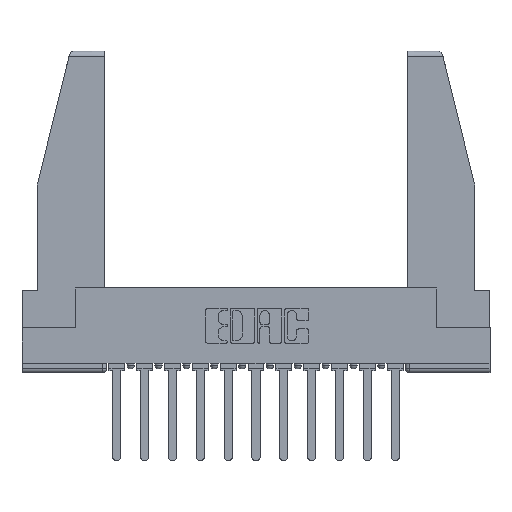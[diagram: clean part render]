
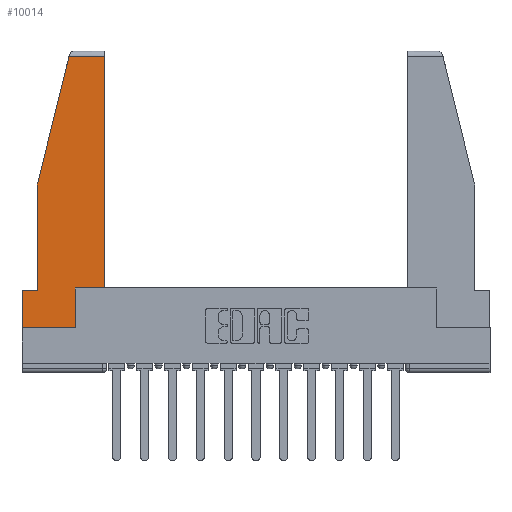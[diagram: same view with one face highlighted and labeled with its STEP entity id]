
A CAD part, top view. The second image highlights one B-rep face of the part: STEP entity #10014.
In plain terms, the highlighted planar face has unit normal (0, 0, 1).
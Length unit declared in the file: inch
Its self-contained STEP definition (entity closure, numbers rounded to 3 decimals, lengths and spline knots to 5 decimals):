
#177 = VERTEX_POINT ( 'NONE', #9312 ) ;
#402 = VECTOR ( 'NONE', #1533, 39.37008 ) ;
#533 = DIRECTION ( 'NONE',  ( -0.239, -0.971, 0. ) ) ;
#787 = CARTESIAN_POINT ( 'NONE',  ( 0.461, 0.223, 0. ) ) ;
#954 = VECTOR ( 'NONE', #12824, 39.37008 ) ;
#1007 = EDGE_CURVE ( 'NONE', #10441, #177, #9274, .T. ) ;
#1317 = CARTESIAN_POINT ( 'NONE',  ( 0.297, 0., 0. ) ) ;
#1343 = CARTESIAN_POINT ( 'NONE',  ( 0.461, 1.52, 0. ) ) ;
#1459 = EDGE_CURVE ( 'NONE', #11042, #12691, #12999, .T. ) ;
#1533 = DIRECTION ( 'NONE',  ( 0., 1., 0. ) ) ;
#1610 = LINE ( 'NONE', #5490, #954 ) ;
#1719 = VERTEX_POINT ( 'NONE', #3285 ) ;
#1766 = CARTESIAN_POINT ( 'NONE',  ( 0.086, 0.8, 0. ) ) ;
#2400 = ORIENTED_EDGE ( 'NONE', *, *, #10114, .T. ) ;
#3152 = CARTESIAN_POINT ( 'NONE',  ( 0., 0.21, 0. ) ) ;
#3285 = CARTESIAN_POINT ( 'NONE',  ( 0.2636, 1.52, 0. ) ) ;
#3377 = CARTESIAN_POINT ( 'NONE',  ( 0., 0., 0. ) ) ;
#3456 = VECTOR ( 'NONE', #4152, 39.37008 ) ;
#3523 = ORIENTED_EDGE ( 'NONE', *, *, #8654, .T. ) ;
#3570 = VECTOR ( 'NONE', #5439, 39.37008 ) ;
#3686 = EDGE_CURVE ( 'NONE', #177, #8543, #5387, .T. ) ;
#3836 = DIRECTION ( 'NONE',  ( 1., 0., 0. ) ) ;
#4152 = DIRECTION ( 'NONE',  ( 0., -1., 0. ) ) ;
#4190 = VECTOR ( 'NONE', #6922, 39.37008 ) ;
#4926 = VERTEX_POINT ( 'NONE', #1343 ) ;
#5168 = CARTESIAN_POINT ( 'NONE',  ( 0.086, 0.21, 0. ) ) ;
#5387 = LINE ( 'NONE', #10444, #12012 ) ;
#5439 = DIRECTION ( 'NONE',  ( 0., -1., 0. ) ) ;
#5490 = CARTESIAN_POINT ( 'NONE',  ( 0., 1.52, 0. ) ) ;
#5506 = CARTESIAN_POINT ( 'NONE',  ( 0., 0.21, 0. ) ) ;
#5519 = LINE ( 'NONE', #13082, #3570 ) ;
#6404 = ORIENTED_EDGE ( 'NONE', *, *, #11941, .T. ) ;
#6805 = ORIENTED_EDGE ( 'NONE', *, *, #7645, .T. ) ;
#6922 = DIRECTION ( 'NONE',  ( 1., 0., 0. ) ) ;
#7645 = EDGE_CURVE ( 'NONE', #13624, #10441, #9221, .T. ) ;
#7898 = DIRECTION ( 'NONE',  ( -1., 0., 0. ) ) ;
#8091 = CARTESIAN_POINT ( 'NONE',  ( 0.297, 0.223, 0. ) ) ;
#8283 = ORIENTED_EDGE ( 'NONE', *, *, #1007, .T. ) ;
#8499 = LINE ( 'NONE', #787, #16318 ) ;
#8543 = VERTEX_POINT ( 'NONE', #1317 ) ;
#8654 = EDGE_CURVE ( 'NONE', #10830, #13624, #5519, .T. ) ;
#8911 = LINE ( 'NONE', #14290, #402 ) ;
#9221 = LINE ( 'NONE', #11646, #9737 ) ;
#9274 = LINE ( 'NONE', #3152, #3456 ) ;
#9312 = CARTESIAN_POINT ( 'NONE',  ( 0., 0., 0. ) ) ;
#9382 = ORIENTED_EDGE ( 'NONE', *, *, #16265, .T. ) ;
#9737 = VECTOR ( 'NONE', #7898, 39.37008 ) ;
#9917 = PLANE ( 'NONE',  #10744 ) ;
#10014 = ADVANCED_FACE ( 'NONE', ( #12240 ), #9917, .T. ) ;
#10114 = EDGE_CURVE ( 'NONE', #12691, #4926, #8499, .T. ) ;
#10441 = VERTEX_POINT ( 'NONE', #5506 ) ;
#10444 = CARTESIAN_POINT ( 'NONE',  ( 0., 0., 0. ) ) ;
#10570 = LINE ( 'NONE', #15647, #15427 ) ;
#10642 = EDGE_CURVE ( 'NONE', #8543, #11042, #8911, .T. ) ;
#10744 = AXIS2_PLACEMENT_3D ( 'NONE', #3377, #14654, #14814 ) ;
#10830 = VERTEX_POINT ( 'NONE', #1766 ) ;
#10906 = DIRECTION ( 'NONE',  ( 0., 1., 0. ) ) ;
#11042 = VERTEX_POINT ( 'NONE', #11386 ) ;
#11386 = CARTESIAN_POINT ( 'NONE',  ( 0.297, 0.223, 0. ) ) ;
#11646 = CARTESIAN_POINT ( 'NONE',  ( 0., 0.21, 0. ) ) ;
#11941 = EDGE_CURVE ( 'NONE', #4926, #1719, #1610, .T. ) ;
#12012 = VECTOR ( 'NONE', #3836, 39.37008 ) ;
#12240 = FACE_OUTER_BOUND ( 'NONE', #15621, .T. ) ;
#12440 = CARTESIAN_POINT ( 'NONE',  ( 0.461, 0.223, 0. ) ) ;
#12454 = ORIENTED_EDGE ( 'NONE', *, *, #3686, .T. ) ;
#12691 = VERTEX_POINT ( 'NONE', #12440 ) ;
#12824 = DIRECTION ( 'NONE',  ( -1., 0., 0. ) ) ;
#12999 = LINE ( 'NONE', #8091, #4190 ) ;
#13082 = CARTESIAN_POINT ( 'NONE',  ( 0.086, 0.8, 0. ) ) ;
#13624 = VERTEX_POINT ( 'NONE', #5168 ) ;
#13724 = ORIENTED_EDGE ( 'NONE', *, *, #10642, .T. ) ;
#14290 = CARTESIAN_POINT ( 'NONE',  ( 0.297, 0., 0. ) ) ;
#14654 = DIRECTION ( 'NONE',  ( 0., 0., 1. ) ) ;
#14814 = DIRECTION ( 'NONE',  ( 1., 0., 0. ) ) ;
#15427 = VECTOR ( 'NONE', #533, 39.37008 ) ;
#15621 = EDGE_LOOP ( 'NONE', ( #2400, #6404, #9382, #3523, #6805, #8283, #12454, #13724, #15936 ) ) ;
#15647 = CARTESIAN_POINT ( 'NONE',  ( 0.271, 1.55, 0. ) ) ;
#15936 = ORIENTED_EDGE ( 'NONE', *, *, #1459, .T. ) ;
#16265 = EDGE_CURVE ( 'NONE', #1719, #10830, #10570, .T. ) ;
#16318 = VECTOR ( 'NONE', #10906, 39.37008 ) ;
